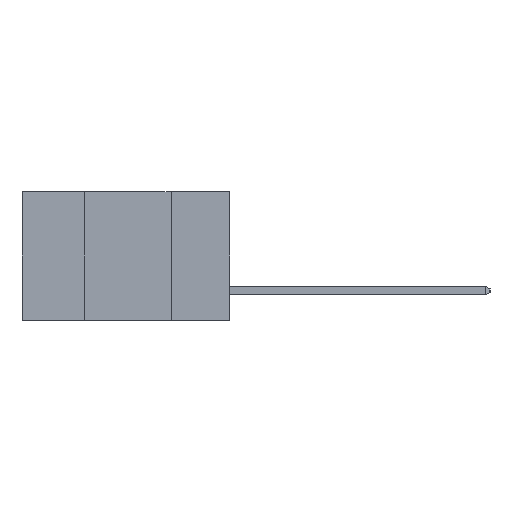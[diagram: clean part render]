
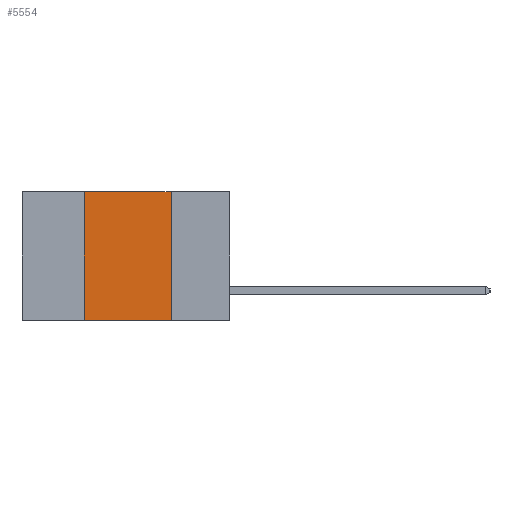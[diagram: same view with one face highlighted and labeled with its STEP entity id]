
A CAD part, left-side view. The second image highlights one B-rep face of the part: STEP entity #5554.
In plain terms, the highlighted planar face has unit normal (-1, 0, 0).
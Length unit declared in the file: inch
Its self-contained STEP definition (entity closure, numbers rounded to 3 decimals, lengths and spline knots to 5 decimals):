
#12 = PLANE ( 'NONE',  #2185 ) ;
#208 = CARTESIAN_POINT ( 'NONE',  ( 0., 0.17, -0.37 ) ) ;
#1141 = ORIENTED_EDGE ( 'NONE', *, *, #10139, .F. ) ;
#1405 = LINE ( 'NONE', #6330, #9448 ) ;
#1578 = DIRECTION ( 'NONE',  ( 0., 0., 1. ) ) ;
#1943 = FACE_OUTER_BOUND ( 'NONE', #11042, .T. ) ;
#1974 = LINE ( 'NONE', #10221, #6552 ) ;
#2150 = DIRECTION ( 'NONE',  ( 1., 0., 0. ) ) ;
#2185 = AXIS2_PLACEMENT_3D ( 'NONE', #7920, #2150, #8870 ) ;
#2543 = CARTESIAN_POINT ( 'NONE',  ( 0., 0.6, 0. ) ) ;
#5372 = DIRECTION ( 'NONE',  ( 0., 0., -1. ) ) ;
#5554 = ADVANCED_FACE ( 'NONE', ( #1943 ), #12, .F. ) ;
#5886 = CARTESIAN_POINT ( 'NONE',  ( 0., 0.42, -0.37 ) ) ;
#5916 = LINE ( 'NONE', #7410, #8410 ) ;
#6090 = ORIENTED_EDGE ( 'NONE', *, *, #11379, .F. ) ;
#6330 = CARTESIAN_POINT ( 'NONE',  ( 0., 0.17, -0.37 ) ) ;
#6401 = ORIENTED_EDGE ( 'NONE', *, *, #8855, .T. ) ;
#6552 = VECTOR ( 'NONE', #11165, 39.37008 ) ;
#6609 = VERTEX_POINT ( 'NONE', #5886 ) ;
#7410 = CARTESIAN_POINT ( 'NONE',  ( 0., 0.42, -0.37 ) ) ;
#7482 = VERTEX_POINT ( 'NONE', #208 ) ;
#7920 = CARTESIAN_POINT ( 'NONE',  ( 0., 0.6, 0. ) ) ;
#8410 = VECTOR ( 'NONE', #1578, 39.37008 ) ;
#8577 = ORIENTED_EDGE ( 'NONE', *, *, #10763, .F. ) ;
#8855 = EDGE_CURVE ( 'NONE', #6609, #7482, #1974, .T. ) ;
#8870 = DIRECTION ( 'NONE',  ( 0., 0., -1. ) ) ;
#9448 = VECTOR ( 'NONE', #5372, 39.37008 ) ;
#9451 = VERTEX_POINT ( 'NONE', #11110 ) ;
#10139 = EDGE_CURVE ( 'NONE', #6609, #9451, #5916, .T. ) ;
#10221 = CARTESIAN_POINT ( 'NONE',  ( 0., 0.6, -0.37 ) ) ;
#10305 = VERTEX_POINT ( 'NONE', #10471 ) ;
#10471 = CARTESIAN_POINT ( 'NONE',  ( 0., 0.17, 0. ) ) ;
#10763 = EDGE_CURVE ( 'NONE', #9451, #10305, #11351, .T. ) ;
#11042 = EDGE_LOOP ( 'NONE', ( #6090, #8577, #1141, #6401 ) ) ;
#11067 = VECTOR ( 'NONE', #12055, 39.37008 ) ;
#11110 = CARTESIAN_POINT ( 'NONE',  ( 0., 0.42, 0. ) ) ;
#11165 = DIRECTION ( 'NONE',  ( 0., -1., 0. ) ) ;
#11351 = LINE ( 'NONE', #2543, #11067 ) ;
#11379 = EDGE_CURVE ( 'NONE', #10305, #7482, #1405, .T. ) ;
#12055 = DIRECTION ( 'NONE',  ( 0., -1., 0. ) ) ;
